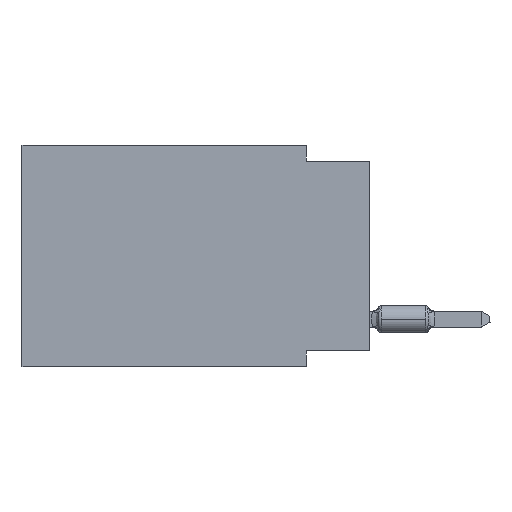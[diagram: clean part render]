
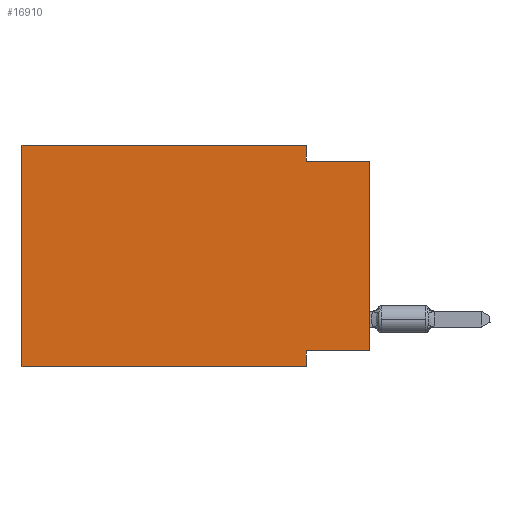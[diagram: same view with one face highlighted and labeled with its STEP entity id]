
A CAD part, left-side view. The second image highlights one B-rep face of the part: STEP entity #16910.
In plain terms, the highlighted planar face has unit normal (-1, 0, 0).
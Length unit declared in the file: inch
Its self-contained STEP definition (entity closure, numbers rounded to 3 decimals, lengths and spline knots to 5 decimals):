
#770 = CARTESIAN_POINT ( 'NONE',  ( 0., 0.55, -0.35 ) ) ;
#992 = VERTEX_POINT ( 'NONE', #21881 ) ;
#1102 = VECTOR ( 'NONE', #4040, 39.37008 ) ;
#1274 = CARTESIAN_POINT ( 'NONE',  ( 0., 0.55, 0. ) ) ;
#1448 = EDGE_CURVE ( 'NONE', #992, #36621, #59407, .T. ) ;
#2277 = CARTESIAN_POINT ( 'NONE',  ( 0., 0., -0.025 ) ) ;
#2424 = CARTESIAN_POINT ( 'NONE',  ( 0., 0., -0.325 ) ) ;
#4040 = DIRECTION ( 'NONE',  ( 0., 0., 1. ) ) ;
#5771 = CARTESIAN_POINT ( 'NONE',  ( 0., 0.1, 0. ) ) ;
#7260 = VERTEX_POINT ( 'NONE', #14081 ) ;
#7394 = VERTEX_POINT ( 'NONE', #39416 ) ;
#9267 = EDGE_LOOP ( 'NONE', ( #56320, #13438, #25234, #34997, #10035, #19971, #63147, #13242 ) ) ;
#10035 = ORIENTED_EDGE ( 'NONE', *, *, #18151, .F. ) ;
#11168 = CARTESIAN_POINT ( 'NONE',  ( 0., 0.1, -0.35 ) ) ;
#12580 = DIRECTION ( 'NONE',  ( 0., 0., 1. ) ) ;
#13242 = ORIENTED_EDGE ( 'NONE', *, *, #50741, .F. ) ;
#13438 = ORIENTED_EDGE ( 'NONE', *, *, #54253, .F. ) ;
#14081 = CARTESIAN_POINT ( 'NONE',  ( 0., 0.55, 0. ) ) ;
#16910 = ADVANCED_FACE ( 'NONE', ( #67487 ), #20518, .F. ) ;
#18151 = EDGE_CURVE ( 'NONE', #992, #7260, #43476, .T. ) ;
#18325 = LINE ( 'NONE', #66658, #56209 ) ;
#18646 = EDGE_CURVE ( 'NONE', #39128, #7394, #18325, .T. ) ;
#19215 = CARTESIAN_POINT ( 'NONE',  ( 0., 0.1, -0.325 ) ) ;
#19971 = ORIENTED_EDGE ( 'NONE', *, *, #1448, .T. ) ;
#20518 = PLANE ( 'NONE',  #33290 ) ;
#21039 = VERTEX_POINT ( 'NONE', #2277 ) ;
#21881 = CARTESIAN_POINT ( 'NONE',  ( 0., 0.55, -0.35 ) ) ;
#25234 = ORIENTED_EDGE ( 'NONE', *, *, #18646, .F. ) ;
#27410 = VERTEX_POINT ( 'NONE', #19215 ) ;
#27768 = CARTESIAN_POINT ( 'NONE',  ( 0., 0., -0.025 ) ) ;
#29143 = VERTEX_POINT ( 'NONE', #2424 ) ;
#31496 = CARTESIAN_POINT ( 'NONE',  ( 0., 0.55, 0. ) ) ;
#32268 = LINE ( 'NONE', #27768, #43080 ) ;
#32867 = VECTOR ( 'NONE', #64548, 39.37008 ) ;
#33290 = AXIS2_PLACEMENT_3D ( 'NONE', #31496, #52406, #42142 ) ;
#34997 = ORIENTED_EDGE ( 'NONE', *, *, #41614, .F. ) ;
#35285 = CARTESIAN_POINT ( 'NONE',  ( 0., 0., 0. ) ) ;
#36621 = VERTEX_POINT ( 'NONE', #62349 ) ;
#39128 = VERTEX_POINT ( 'NONE', #5771 ) ;
#39416 = CARTESIAN_POINT ( 'NONE',  ( 0., 0.1, -0.025 ) ) ;
#40437 = LINE ( 'NONE', #35285, #1102 ) ;
#40572 = VECTOR ( 'NONE', #52566, 39.37008 ) ;
#41614 = EDGE_CURVE ( 'NONE', #7260, #39128, #47647, .T. ) ;
#42142 = DIRECTION ( 'NONE',  ( 0., 0., -1. ) ) ;
#43080 = VECTOR ( 'NONE', #53170, 39.37008 ) ;
#43476 = LINE ( 'NONE', #1274, #64968 ) ;
#47647 = LINE ( 'NONE', #54116, #51509 ) ;
#50587 = DIRECTION ( 'NONE',  ( 0., 0., -1. ) ) ;
#50741 = EDGE_CURVE ( 'NONE', #29143, #27410, #53898, .T. ) ;
#51509 = VECTOR ( 'NONE', #57916, 39.37008 ) ;
#51902 = VECTOR ( 'NONE', #53344, 39.37008 ) ;
#52406 = DIRECTION ( 'NONE',  ( 1., 0., 0. ) ) ;
#52566 = DIRECTION ( 'NONE',  ( 0., 1., 0. ) ) ;
#52900 = CARTESIAN_POINT ( 'NONE',  ( 0., 0., -0.325 ) ) ;
#53170 = DIRECTION ( 'NONE',  ( 0., -1., 0. ) ) ;
#53344 = DIRECTION ( 'NONE',  ( 0., 0., -1. ) ) ;
#53898 = LINE ( 'NONE', #52900, #40572 ) ;
#54116 = CARTESIAN_POINT ( 'NONE',  ( 0., 0.55, 0. ) ) ;
#54253 = EDGE_CURVE ( 'NONE', #7394, #21039, #32268, .T. ) ;
#56209 = VECTOR ( 'NONE', #50587, 39.37008 ) ;
#56320 = ORIENTED_EDGE ( 'NONE', *, *, #65923, .T. ) ;
#56792 = EDGE_CURVE ( 'NONE', #27410, #36621, #58819, .T. ) ;
#57916 = DIRECTION ( 'NONE',  ( 0., -1., 0. ) ) ;
#58819 = LINE ( 'NONE', #11168, #51902 ) ;
#59407 = LINE ( 'NONE', #770, #32867 ) ;
#62349 = CARTESIAN_POINT ( 'NONE',  ( 0., 0.1, -0.35 ) ) ;
#63147 = ORIENTED_EDGE ( 'NONE', *, *, #56792, .F. ) ;
#64548 = DIRECTION ( 'NONE',  ( 0., -1., 0. ) ) ;
#64968 = VECTOR ( 'NONE', #12580, 39.37008 ) ;
#65923 = EDGE_CURVE ( 'NONE', #29143, #21039, #40437, .T. ) ;
#66658 = CARTESIAN_POINT ( 'NONE',  ( 0., 0.1, 0. ) ) ;
#67487 = FACE_OUTER_BOUND ( 'NONE', #9267, .T. ) ;
